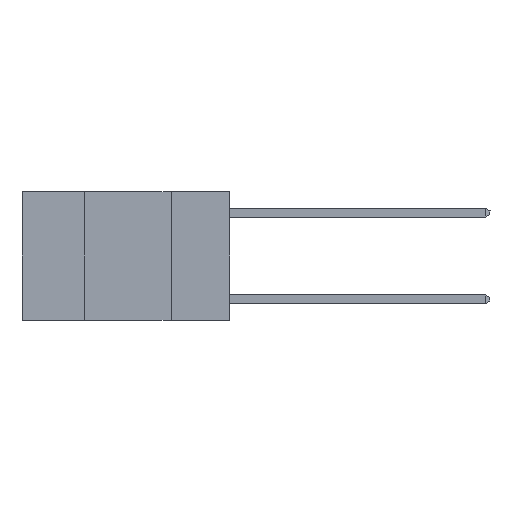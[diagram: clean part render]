
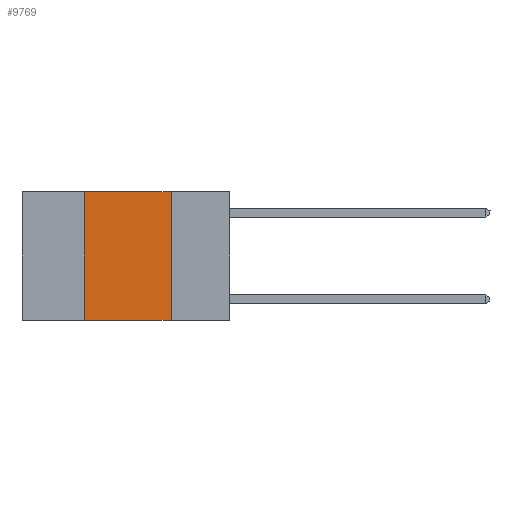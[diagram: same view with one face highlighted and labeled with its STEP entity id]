
A CAD part, left-side view. The second image highlights one B-rep face of the part: STEP entity #9769.
In plain terms, the highlighted planar face has unit normal (-1, 0, 0).
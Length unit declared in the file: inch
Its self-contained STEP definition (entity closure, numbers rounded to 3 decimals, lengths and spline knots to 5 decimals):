
#36 = DIRECTION ( 'NONE',  ( 1., 0., 0. ) ) ;
#868 = VERTEX_POINT ( 'NONE', #2336 ) ;
#917 = LINE ( 'NONE', #5264, #13076 ) ;
#921 = EDGE_CURVE ( 'NONE', #13447, #868, #917, .T. ) ;
#1399 = FACE_OUTER_BOUND ( 'NONE', #2154, .T. ) ;
#2154 = EDGE_LOOP ( 'NONE', ( #19436, #7157, #11915, #3368 ) ) ;
#2336 = CARTESIAN_POINT ( 'NONE',  ( 0., 0.17, 0. ) ) ;
#3368 = ORIENTED_EDGE ( 'NONE', *, *, #17082, .T. ) ;
#4452 = CARTESIAN_POINT ( 'NONE',  ( 0., 0.42, 0. ) ) ;
#4546 = LINE ( 'NONE', #9089, #8138 ) ;
#4884 = EDGE_CURVE ( 'NONE', #868, #9323, #19030, .T. ) ;
#5264 = CARTESIAN_POINT ( 'NONE',  ( 0., 0.6, 0. ) ) ;
#6047 = DIRECTION ( 'NONE',  ( 0., 0., -1. ) ) ;
#7157 = ORIENTED_EDGE ( 'NONE', *, *, #921, .F. ) ;
#7331 = DIRECTION ( 'NONE',  ( 0., 0., -1. ) ) ;
#7442 = PLANE ( 'NONE',  #10891 ) ;
#8000 = CARTESIAN_POINT ( 'NONE',  ( 0., 0.42, 0. ) ) ;
#8138 = VECTOR ( 'NONE', #10754, 39.37008 ) ;
#9089 = CARTESIAN_POINT ( 'NONE',  ( 0., 0.6, -0.37 ) ) ;
#9108 = CARTESIAN_POINT ( 'NONE',  ( 0., 0.42, -0.37 ) ) ;
#9275 = DIRECTION ( 'NONE',  ( 0., 0., 1. ) ) ;
#9323 = VERTEX_POINT ( 'NONE', #19185 ) ;
#9769 = ADVANCED_FACE ( 'NONE', ( #1399 ), #7442, .F. ) ;
#9879 = VERTEX_POINT ( 'NONE', #9108 ) ;
#10077 = DIRECTION ( 'NONE',  ( 0., -1., 0. ) ) ;
#10754 = DIRECTION ( 'NONE',  ( 0., -1., 0. ) ) ;
#10891 = AXIS2_PLACEMENT_3D ( 'NONE', #13527, #36, #6047 ) ;
#11915 = ORIENTED_EDGE ( 'NONE', *, *, #18510, .F. ) ;
#12245 = LINE ( 'NONE', #4452, #16673 ) ;
#13076 = VECTOR ( 'NONE', #10077, 39.37008 ) ;
#13447 = VERTEX_POINT ( 'NONE', #8000 ) ;
#13527 = CARTESIAN_POINT ( 'NONE',  ( 0., 0.6, 0. ) ) ;
#16161 = VECTOR ( 'NONE', #7331, 39.37008 ) ;
#16673 = VECTOR ( 'NONE', #9275, 39.37008 ) ;
#17082 = EDGE_CURVE ( 'NONE', #9879, #9323, #4546, .T. ) ;
#17568 = CARTESIAN_POINT ( 'NONE',  ( 0., 0.17, 0. ) ) ;
#18510 = EDGE_CURVE ( 'NONE', #9879, #13447, #12245, .T. ) ;
#19030 = LINE ( 'NONE', #17568, #16161 ) ;
#19185 = CARTESIAN_POINT ( 'NONE',  ( 0., 0.17, -0.37 ) ) ;
#19436 = ORIENTED_EDGE ( 'NONE', *, *, #4884, .F. ) ;
